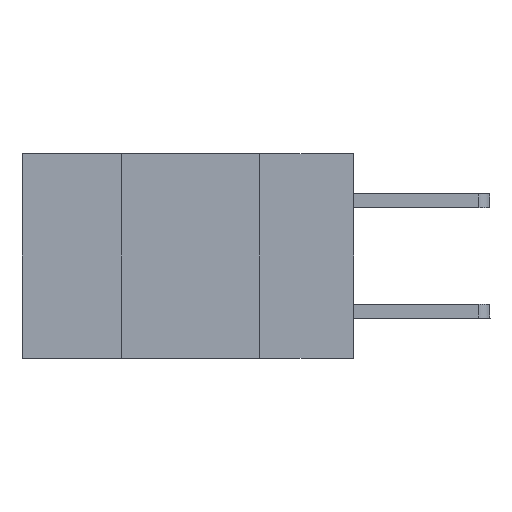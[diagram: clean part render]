
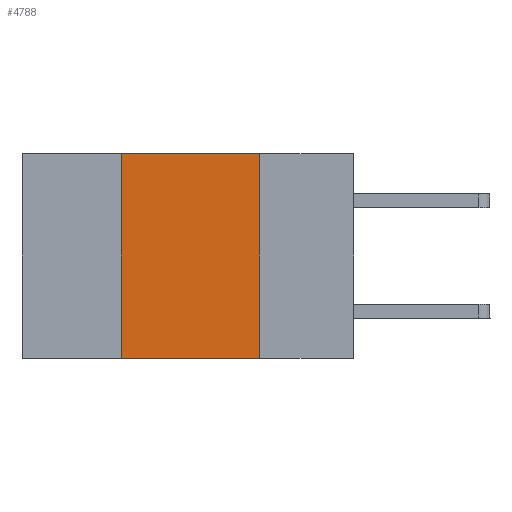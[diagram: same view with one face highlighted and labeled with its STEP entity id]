
A CAD part, left-side view. The second image highlights one B-rep face of the part: STEP entity #4788.
In plain terms, the highlighted planar face has unit normal (-1, 0, 0).
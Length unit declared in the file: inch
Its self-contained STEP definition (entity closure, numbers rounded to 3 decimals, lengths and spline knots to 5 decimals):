
#422 = VERTEX_POINT ( 'NONE', #8978 ) ;
#1104 = VERTEX_POINT ( 'NONE', #8578 ) ;
#1111 = CARTESIAN_POINT ( 'NONE',  ( 0., 0.17, 0. ) ) ;
#1405 = CARTESIAN_POINT ( 'NONE',  ( 0., 0.42, 0. ) ) ;
#1966 = VERTEX_POINT ( 'NONE', #1111 ) ;
#1984 = ORIENTED_EDGE ( 'NONE', *, *, #9580, .F. ) ;
#2192 = FACE_OUTER_BOUND ( 'NONE', #2943, .T. ) ;
#2287 = CARTESIAN_POINT ( 'NONE',  ( 0., 0.17, 0. ) ) ;
#2325 = DIRECTION ( 'NONE',  ( 0., 0., -1. ) ) ;
#2568 = ORIENTED_EDGE ( 'NONE', *, *, #6243, .F. ) ;
#2685 = CARTESIAN_POINT ( 'NONE',  ( 0., 0.42, 0. ) ) ;
#2770 = PLANE ( 'NONE',  #10796 ) ;
#2943 = EDGE_LOOP ( 'NONE', ( #1984, #2568, #10140, #5107 ) ) ;
#3839 = LINE ( 'NONE', #5250, #10507 ) ;
#4180 = VECTOR ( 'NONE', #10105, 39.37008 ) ;
#4704 = DIRECTION ( 'NONE',  ( 0., 0., 1. ) ) ;
#4760 = LINE ( 'NONE', #1405, #7182 ) ;
#4788 = ADVANCED_FACE ( 'NONE', ( #2192 ), #2770, .F. ) ;
#5107 = ORIENTED_EDGE ( 'NONE', *, *, #7224, .T. ) ;
#5201 = EDGE_CURVE ( 'NONE', #422, #9245, #4760, .T. ) ;
#5250 = CARTESIAN_POINT ( 'NONE',  ( 0., 0.6, 0. ) ) ;
#5742 = CARTESIAN_POINT ( 'NONE',  ( 0., 0.6, 0. ) ) ;
#6243 = EDGE_CURVE ( 'NONE', #9245, #1966, #3839, .T. ) ;
#6339 = VECTOR ( 'NONE', #2325, 39.37008 ) ;
#6749 = CARTESIAN_POINT ( 'NONE',  ( 0., 0.6, -0.37 ) ) ;
#7182 = VECTOR ( 'NONE', #4704, 39.37008 ) ;
#7224 = EDGE_CURVE ( 'NONE', #422, #1104, #8940, .T. ) ;
#7450 = DIRECTION ( 'NONE',  ( 0., 0., -1. ) ) ;
#8578 = CARTESIAN_POINT ( 'NONE',  ( 0., 0.17, -0.37 ) ) ;
#8657 = LINE ( 'NONE', #2287, #6339 ) ;
#8940 = LINE ( 'NONE', #6749, #4180 ) ;
#8978 = CARTESIAN_POINT ( 'NONE',  ( 0., 0.42, -0.37 ) ) ;
#9245 = VERTEX_POINT ( 'NONE', #2685 ) ;
#9541 = DIRECTION ( 'NONE',  ( 0., -1., 0. ) ) ;
#9580 = EDGE_CURVE ( 'NONE', #1966, #1104, #8657, .T. ) ;
#9809 = DIRECTION ( 'NONE',  ( 1., 0., 0. ) ) ;
#10105 = DIRECTION ( 'NONE',  ( 0., -1., 0. ) ) ;
#10140 = ORIENTED_EDGE ( 'NONE', *, *, #5201, .F. ) ;
#10507 = VECTOR ( 'NONE', #9541, 39.37008 ) ;
#10796 = AXIS2_PLACEMENT_3D ( 'NONE', #5742, #9809, #7450 ) ;
